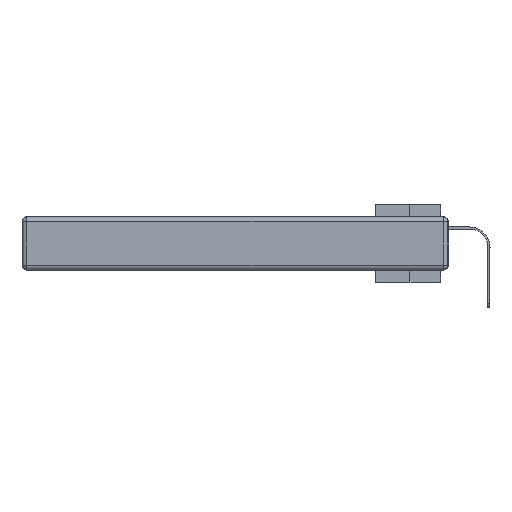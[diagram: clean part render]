
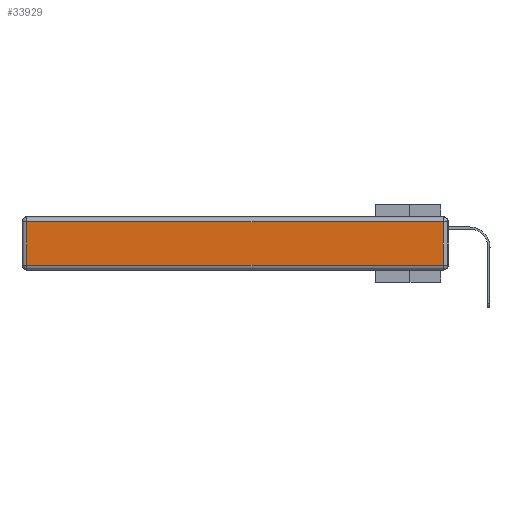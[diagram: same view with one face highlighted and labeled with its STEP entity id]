
A CAD part, left-side view. The second image highlights one B-rep face of the part: STEP entity #33929.
In plain terms, the highlighted planar face has unit normal (-1, 0, 0).
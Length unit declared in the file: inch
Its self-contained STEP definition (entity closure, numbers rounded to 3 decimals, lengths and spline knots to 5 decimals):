
#575 = CARTESIAN_POINT ( 'NONE',  ( 0., 2.72, -0.343 ) ) ;
#3752 = CARTESIAN_POINT ( 'NONE',  ( 0., 2.72, -0.03 ) ) ;
#3767 = EDGE_CURVE ( 'NONE', #33226, #19753, #25522, .T. ) ;
#3849 = DIRECTION ( 'NONE',  ( -1., 0., 0. ) ) ;
#4020 = DIRECTION ( 'NONE',  ( 0., 1., 0. ) ) ;
#4304 = ORIENTED_EDGE ( 'NONE', *, *, #18243, .T. ) ;
#4921 = CARTESIAN_POINT ( 'NONE',  ( 0., 0.03, -0.343 ) ) ;
#5928 = LINE ( 'NONE', #575, #11058 ) ;
#6156 = VECTOR ( 'NONE', #34470, 39.37008 ) ;
#6972 = VERTEX_POINT ( 'NONE', #28292 ) ;
#7244 = CARTESIAN_POINT ( 'NONE',  ( 0., 0., -0.313 ) ) ;
#9307 = ORIENTED_EDGE ( 'NONE', *, *, #3767, .T. ) ;
#9370 = CARTESIAN_POINT ( 'NONE',  ( 0., 0., -0.343 ) ) ;
#9634 = EDGE_CURVE ( 'NONE', #17882, #6972, #34298, .T. ) ;
#11058 = VECTOR ( 'NONE', #27797, 39.37008 ) ;
#12552 = VECTOR ( 'NONE', #18219, 39.37008 ) ;
#12607 = ORIENTED_EDGE ( 'NONE', *, *, #17591, .T. ) ;
#13958 = CARTESIAN_POINT ( 'NONE',  ( 0., 2.72, -0.313 ) ) ;
#14855 = DIRECTION ( 'NONE',  ( 0., 0., 1. ) ) ;
#17591 = EDGE_CURVE ( 'NONE', #6972, #33226, #28750, .T. ) ;
#17682 = FACE_OUTER_BOUND ( 'NONE', #18797, .T. ) ;
#17882 = VERTEX_POINT ( 'NONE', #13958 ) ;
#18219 = DIRECTION ( 'NONE',  ( 0., 0., 1. ) ) ;
#18243 = EDGE_CURVE ( 'NONE', #19753, #17882, #5928, .T. ) ;
#18797 = EDGE_LOOP ( 'NONE', ( #32619, #12607, #9307, #4304 ) ) ;
#19753 = VERTEX_POINT ( 'NONE', #3752 ) ;
#21329 = CARTESIAN_POINT ( 'NONE',  ( 0., 0.03, -0.03 ) ) ;
#22868 = PLANE ( 'NONE',  #27507 ) ;
#24268 = VECTOR ( 'NONE', #4020, 39.37008 ) ;
#25522 = LINE ( 'NONE', #28026, #24268 ) ;
#27507 = AXIS2_PLACEMENT_3D ( 'NONE', #9370, #3849, #14855 ) ;
#27797 = DIRECTION ( 'NONE',  ( 0., 0., -1. ) ) ;
#28026 = CARTESIAN_POINT ( 'NONE',  ( 0., 2.75, -0.03 ) ) ;
#28292 = CARTESIAN_POINT ( 'NONE',  ( 0., 0.03, -0.313 ) ) ;
#28750 = LINE ( 'NONE', #4921, #12552 ) ;
#32619 = ORIENTED_EDGE ( 'NONE', *, *, #9634, .T. ) ;
#33226 = VERTEX_POINT ( 'NONE', #21329 ) ;
#33929 = ADVANCED_FACE ( 'NONE', ( #17682 ), #22868, .T. ) ;
#34298 = LINE ( 'NONE', #7244, #6156 ) ;
#34470 = DIRECTION ( 'NONE',  ( 0., -1., 0. ) ) ;
